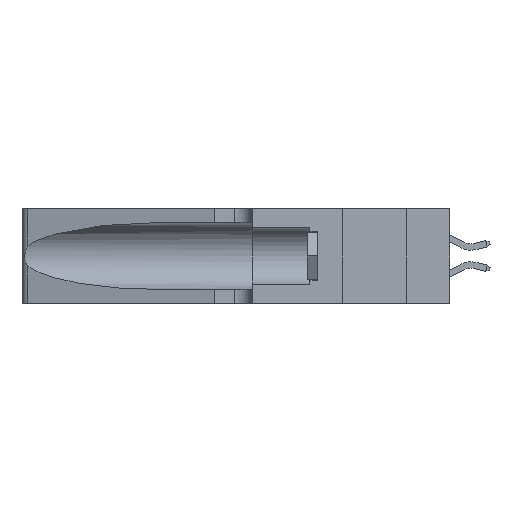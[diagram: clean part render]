
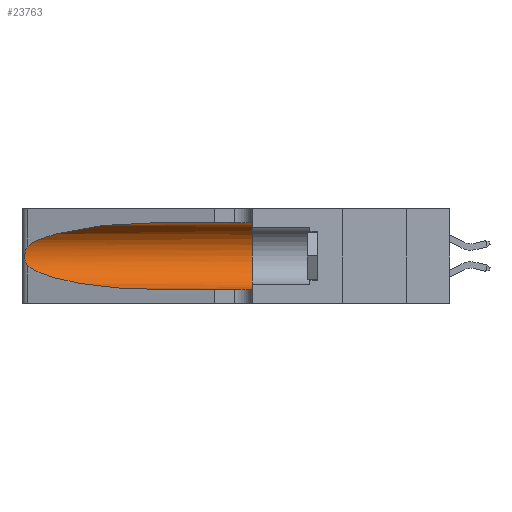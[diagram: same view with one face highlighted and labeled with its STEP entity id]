
A CAD part, left-side view. The second image highlights one B-rep face of the part: STEP entity #23763.
In plain terms, the highlighted cylindrical face has radius 3.308 mm (diameter 6.617 mm), a partial arc.
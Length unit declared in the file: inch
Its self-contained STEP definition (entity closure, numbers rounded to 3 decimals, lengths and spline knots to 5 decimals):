
#224 =( BOUNDED_CURVE ( )  B_SPLINE_CURVE ( 3, ( #6366, #19991, #9867, #33479 ),
 .UNSPECIFIED., .F., .T. ) 
 B_SPLINE_CURVE_WITH_KNOTS ( ( 4, 4 ),
 ( 3.44316, 4.71239 ),
 .UNSPECIFIED. ) 
 CURVE ( )  GEOMETRIC_REPRESENTATION_ITEM ( )  RATIONAL_B_SPLINE_CURVE ( ( 1., 0.87, 0.87, 1. ) ) 
 REPRESENTATION_ITEM ( '' )  );
#595 = ORIENTED_EDGE ( 'NONE', *, *, #13342, .T. ) ;
#2267 = VECTOR ( 'NONE', #34084, 39.37008 ) ;
#2646 = CARTESIAN_POINT ( 'NONE',  ( 0.25555, 1.22994, 0.2215 ) ) ;
#3294 = DIRECTION ( 'NONE',  ( 0., 0., 1. ) ) ;
#3369 = CIRCLE ( 'NONE', #13544, 0.13025 ) ;
#4085 = EDGE_LOOP ( 'NONE', ( #595, #36804, #35072, #7277, #20421, #15694 ) ) ;
#6109 = CARTESIAN_POINT ( 'NONE',  ( 0.25787, 1.23484, 0.2124 ) ) ;
#6366 = CARTESIAN_POINT ( 'NONE',  ( 0.25487, 1.22718, 0.14631 ) ) ;
#6428 = CARTESIAN_POINT ( 'NONE',  ( 0.1305, 1.61858, 0.31525 ) ) ;
#6903 = VERTEX_POINT ( 'NONE', #42275 ) ;
#7154 = VERTEX_POINT ( 'NONE', #26662 ) ;
#7277 = ORIENTED_EDGE ( 'NONE', *, *, #34013, .T. ) ;
#8731 = CARTESIAN_POINT ( 'NONE',  ( 0.18966, 0.96281, 0.31525 ) ) ;
#9603 = CARTESIAN_POINT ( 'NONE',  ( 0.26018, 1.23835, 0.19895 ) ) ;
#9867 = CARTESIAN_POINT ( 'NONE',  ( 0.18966, 0.96281, 0.05475 ) ) ;
#11430 = AXIS2_PLACEMENT_3D ( 'NONE', #35436, #11841, #42045 ) ;
#11841 = DIRECTION ( 'NONE',  ( 0., -1., 0. ) ) ;
#12197 = CARTESIAN_POINT ( 'NONE',  ( 0.1305, 0.72297, 0.31525 ) ) ;
#13063 = CARTESIAN_POINT ( 'NONE',  ( 0.26075, 1.23896, 0.178 ) ) ;
#13342 = EDGE_CURVE ( 'NONE', #37471, #42929, #16298, .T. ) ;
#13544 = AXIS2_PLACEMENT_3D ( 'NONE', #43829, #23689, #3294 ) ;
#15284 = VERTEX_POINT ( 'NONE', #22233 ) ;
#15642 = CARTESIAN_POINT ( 'NONE',  ( 0.25487, 1.22718, 0.22369 ) ) ;
#15694 = ORIENTED_EDGE ( 'NONE', *, *, #31541, .F. ) ;
#16298 =( BOUNDED_CURVE ( )  B_SPLINE_CURVE ( 3, ( #12197, #8731, #29015, #15642 ),
 .UNSPECIFIED., .F., .F. ) 
 B_SPLINE_CURVE_WITH_KNOTS ( ( 4, 4 ),
 ( 1.5708, 2.84003 ),
 .UNSPECIFIED. ) 
 CURVE ( )  GEOMETRIC_REPRESENTATION_ITEM ( )  RATIONAL_B_SPLINE_CURVE ( ( 1., 0.87, 0.87, 1. ) ) 
 REPRESENTATION_ITEM ( '' )  );
#16481 = CARTESIAN_POINT ( 'NONE',  ( 0.25856, 1.23593, 0.16098 ) ) ;
#18779 = FACE_OUTER_BOUND ( 'NONE', #4085, .T. ) ;
#18856 = VECTOR ( 'NONE', #33546, 39.37008 ) ;
#19887 = CARTESIAN_POINT ( 'NONE',  ( 0.25639, 1.23186, 0.15144 ) ) ;
#19991 = CARTESIAN_POINT ( 'NONE',  ( 0.2373, 1.15595, 0.08982 ) ) ;
#20421 = ORIENTED_EDGE ( 'NONE', *, *, #27439, .F. ) ;
#20469 = EDGE_CURVE ( 'NONE', #6903, #15284, #224, .T. ) ;
#22233 = CARTESIAN_POINT ( 'NONE',  ( 0.1305, 0.72297, 0.05475 ) ) ;
#23004 = CARTESIAN_POINT ( 'NONE',  ( 0.1305, 0.72297, 0.31525 ) ) ;
#23023 = LINE ( 'NONE', #6428, #18856 ) ;
#23219 = CARTESIAN_POINT ( 'NONE',  ( 0.25487, 1.22718, 0.14631 ) ) ;
#23689 = DIRECTION ( 'NONE',  ( 0., 1., 0. ) ) ;
#23763 = ADVANCED_FACE ( 'NONE', ( #18779 ), #35572, .F. ) ;
#26450 = CARTESIAN_POINT ( 'NONE',  ( 0.25639, 1.23184, 0.21858 ) ) ;
#26662 = CARTESIAN_POINT ( 'NONE',  ( 0.1305, 0.35, 0.31525 ) ) ;
#27439 = EDGE_CURVE ( 'NONE', #7154, #31629, #3369, .T. ) ;
#28866 = EDGE_CURVE ( 'NONE', #42929, #6903, #33229, .T. ) ;
#29015 = CARTESIAN_POINT ( 'NONE',  ( 0.2373, 1.15595, 0.28018 ) ) ;
#29415 = LINE ( 'NONE', #37452, #2267 ) ;
#29843 = CARTESIAN_POINT ( 'NONE',  ( 0.25854, 1.2359, 0.20912 ) ) ;
#30579 = CARTESIAN_POINT ( 'NONE',  ( 0.1305, 0.35, 0.05475 ) ) ;
#31541 = EDGE_CURVE ( 'NONE', #37471, #7154, #23023, .T. ) ;
#31629 = VERTEX_POINT ( 'NONE', #30579 ) ;
#33220 = CARTESIAN_POINT ( 'NONE',  ( 0.26075, 1.23896, 0.19203 ) ) ;
#33229 = B_SPLINE_CURVE_WITH_KNOTS ( 'NONE', 3,
 ( #43208, #2646, #26450, #6109, #29843, #9603, #33220, #13063, #36609, #16481, #40002, #19887, #43350, #23219 ),
 .UNSPECIFIED., .F., .F.,
 ( 4, 2, 2, 2, 2, 2, 4 ),
 ( 0., 0.00027, 0.00053, 0.00107, 0.0016, 0.00187, 0.00214 ),
 .UNSPECIFIED. ) ;
#33479 = CARTESIAN_POINT ( 'NONE',  ( 0.1305, 0.72297, 0.05475 ) ) ;
#33546 = DIRECTION ( 'NONE',  ( 0., -1., 0. ) ) ;
#34013 = EDGE_CURVE ( 'NONE', #15284, #31629, #29415, .T. ) ;
#34084 = DIRECTION ( 'NONE',  ( 0., -1., 0. ) ) ;
#35072 = ORIENTED_EDGE ( 'NONE', *, *, #20469, .T. ) ;
#35436 = CARTESIAN_POINT ( 'NONE',  ( 0.1305, 1.61858, 0.185 ) ) ;
#35572 = CYLINDRICAL_SURFACE ( 'NONE', #11430, 0.13025 ) ;
#36609 = CARTESIAN_POINT ( 'NONE',  ( 0.26017, 1.23833, 0.17102 ) ) ;
#36804 = ORIENTED_EDGE ( 'NONE', *, *, #28866, .T. ) ;
#37452 = CARTESIAN_POINT ( 'NONE',  ( 0.1305, 1.61858, 0.05475 ) ) ;
#37471 = VERTEX_POINT ( 'NONE', #23004 ) ;
#38117 = CARTESIAN_POINT ( 'NONE',  ( 0.25487, 1.22718, 0.22369 ) ) ;
#40002 = CARTESIAN_POINT ( 'NONE',  ( 0.25789, 1.23486, 0.15765 ) ) ;
#42045 = DIRECTION ( 'NONE',  ( 0., 0., -1. ) ) ;
#42275 = CARTESIAN_POINT ( 'NONE',  ( 0.25487, 1.22718, 0.14631 ) ) ;
#42929 = VERTEX_POINT ( 'NONE', #38117 ) ;
#43208 = CARTESIAN_POINT ( 'NONE',  ( 0.25487, 1.22718, 0.22369 ) ) ;
#43350 = CARTESIAN_POINT ( 'NONE',  ( 0.25555, 1.22993, 0.14849 ) ) ;
#43829 = CARTESIAN_POINT ( 'NONE',  ( 0.1305, 0.35, 0.185 ) ) ;
